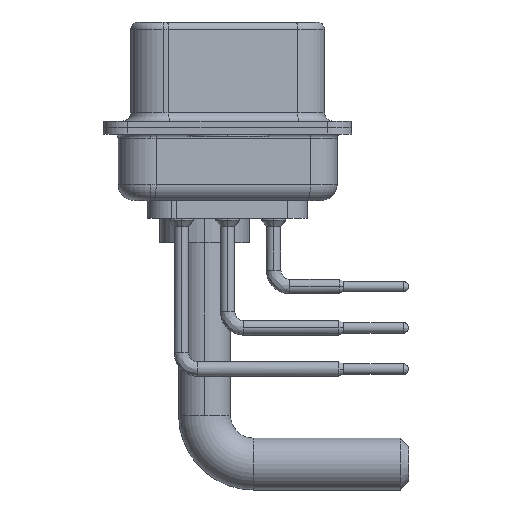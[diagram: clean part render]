
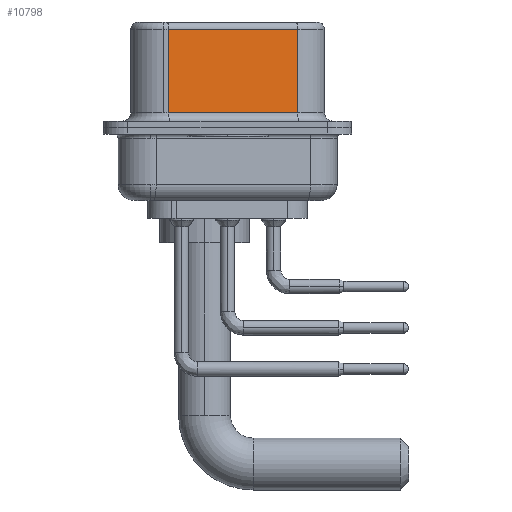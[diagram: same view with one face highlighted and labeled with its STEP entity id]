
A CAD part, left-side view. The second image highlights one B-rep face of the part: STEP entity #10798.
In plain terms, the highlighted planar face has unit normal (-0.985, -0.174, 0).
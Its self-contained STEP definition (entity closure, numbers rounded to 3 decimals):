
#1422 = CARTESIAN_POINT ( 'NONE',  ( 5.132, -4.322, 6.02 ) ) ;
#3248 = LINE ( 'NONE', #11535, #25974 ) ;
#3421 = DIRECTION ( 'NONE',  ( 0., 0., -1. ) ) ;
#3468 = VECTOR ( 'NONE', #3421, 1000. ) ;
#4218 = VERTEX_POINT ( 'NONE', #1422 ) ;
#6727 = ORIENTED_EDGE ( 'NONE', *, *, #15897, .T. ) ;
#7131 = CARTESIAN_POINT ( 'NONE',  ( 5.132, -4.322, 6.02 ) ) ;
#7457 = DIRECTION ( 'NONE',  ( 0., 0., -1. ) ) ;
#8626 = PLANE ( 'NONE',  #19423 ) ;
#9313 = CARTESIAN_POINT ( 'NONE',  ( 3.73, 3.628, 0.9 ) ) ;
#9831 = DIRECTION ( 'NONE',  ( -0.174, 0.985, 0. ) ) ;
#10143 = EDGE_CURVE ( 'NONE', #4218, #18880, #15050, .T. ) ;
#10798 = ADVANCED_FACE ( 'NONE', ( #19643 ), #8626, .F. ) ;
#11321 = DIRECTION ( 'NONE',  ( -0.174, 0.985, 0. ) ) ;
#11392 = VECTOR ( 'NONE', #9831, 1000. ) ;
#11535 = CARTESIAN_POINT ( 'NONE',  ( 5.132, -4.322, 0.9 ) ) ;
#14901 = LINE ( 'NONE', #7131, #11392 ) ;
#15050 = LINE ( 'NONE', #28734, #19455 ) ;
#15302 = VERTEX_POINT ( 'NONE', #30768 ) ;
#15897 = EDGE_CURVE ( 'NONE', #4218, #15302, #14901, .T. ) ;
#18880 = VERTEX_POINT ( 'NONE', #24080 ) ;
#19106 = CARTESIAN_POINT ( 'NONE',  ( 5.132, -4.322, 6.52 ) ) ;
#19423 = AXIS2_PLACEMENT_3D ( 'NONE', #19106, #24675, #11321 ) ;
#19455 = VECTOR ( 'NONE', #7457, 1000. ) ;
#19643 = FACE_OUTER_BOUND ( 'NONE', #25761, .T. ) ;
#20229 = EDGE_CURVE ( 'NONE', #31146, #18880, #3248, .T. ) ;
#23149 = ORIENTED_EDGE ( 'NONE', *, *, #20229, .T. ) ;
#24080 = CARTESIAN_POINT ( 'NONE',  ( 5.132, -4.322, 0.9 ) ) ;
#24675 = DIRECTION ( 'NONE',  ( 0.985, 0.174, 0. ) ) ;
#25761 = EDGE_LOOP ( 'NONE', ( #29968, #6727, #30709, #23149 ) ) ;
#25974 = VECTOR ( 'NONE', #28276, 1000. ) ;
#27737 = CARTESIAN_POINT ( 'NONE',  ( 3.73, 3.628, 6.52 ) ) ;
#28276 = DIRECTION ( 'NONE',  ( 0.174, -0.985, 0. ) ) ;
#28734 = CARTESIAN_POINT ( 'NONE',  ( 5.132, -4.322, 6.52 ) ) ;
#29300 = EDGE_CURVE ( 'NONE', #15302, #31146, #33135, .T. ) ;
#29968 = ORIENTED_EDGE ( 'NONE', *, *, #10143, .F. ) ;
#30709 = ORIENTED_EDGE ( 'NONE', *, *, #29300, .T. ) ;
#30768 = CARTESIAN_POINT ( 'NONE',  ( 3.73, 3.628, 6.02 ) ) ;
#31146 = VERTEX_POINT ( 'NONE', #9313 ) ;
#33135 = LINE ( 'NONE', #27737, #3468 ) ;
